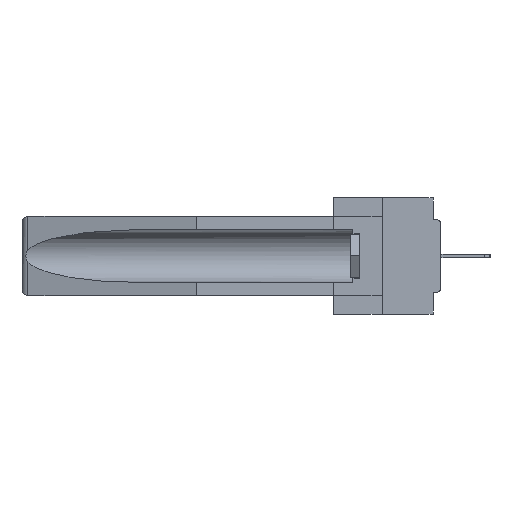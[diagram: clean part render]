
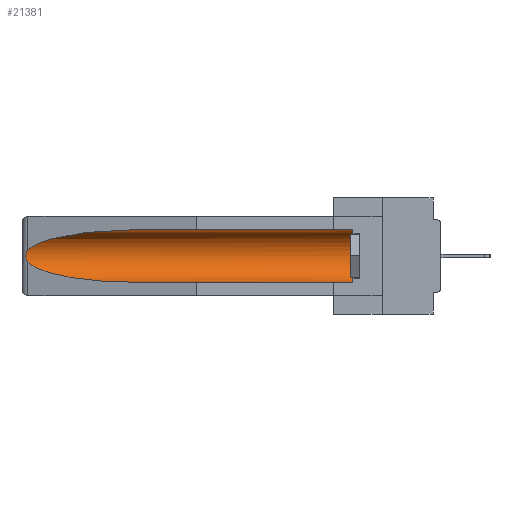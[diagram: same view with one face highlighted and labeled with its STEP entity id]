
A CAD part, left-side view. The second image highlights one B-rep face of the part: STEP entity #21381.
In plain terms, the highlighted cylindrical face has radius 2.857 mm (diameter 5.715 mm), a partial arc.
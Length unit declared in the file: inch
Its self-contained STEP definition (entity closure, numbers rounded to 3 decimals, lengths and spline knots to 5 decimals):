
#842 =( BOUNDED_CURVE ( )  B_SPLINE_CURVE ( 3, ( #7935, #8410, #2810, #5614 ),
 .UNSPECIFIED., .F., .F. ) 
 B_SPLINE_CURVE_WITH_KNOTS ( ( 4, 4 ),
 ( 0.1948, 1.5708 ),
 .UNSPECIFIED. ) 
 CURVE ( )  GEOMETRIC_REPRESENTATION_ITEM ( )  RATIONAL_B_SPLINE_CURVE ( ( 1., 0.848, 0.848, 1. ) ) 
 REPRESENTATION_ITEM ( '' )  );
#1557 = EDGE_CURVE ( 'NONE', #12987, #19888, #22805, .T. ) ;
#1878 = LINE ( 'NONE', #9308, #30999 ) ;
#2533 = CARTESIAN_POINT ( 'NONE',  ( 0.2675, 1.53308, -0.16763 ) ) ;
#2810 = CARTESIAN_POINT ( 'NONE',  ( 0.21114, 1.30732, -0.284 ) ) ;
#3015 = CARTESIAN_POINT ( 'NONE',  ( 0.26597, 1.5296, -0.19026 ) ) ;
#3927 = EDGE_LOOP ( 'NONE', ( #12949, #23673, #14191, #20234, #22389, #15519 ) ) ;
#4644 = EDGE_CURVE ( 'NONE', #16827, #7737, #842, .T. ) ;
#4791 = AXIS2_PLACEMENT_3D ( 'NONE', #25932, #20334, #13155 ) ;
#4849 = CARTESIAN_POINT ( 'NONE',  ( 0.26537, 1.52718, -0.19328 ) ) ;
#5614 = CARTESIAN_POINT ( 'NONE',  ( 0.155, 1.07973, -0.284 ) ) ;
#6526 =( BOUNDED_CURVE ( )  B_SPLINE_CURVE ( 3, ( #12414, #9428, #15060, #25206 ),
 .UNSPECIFIED., .F., .F. ) 
 B_SPLINE_CURVE_WITH_KNOTS ( ( 4, 4 ),
 ( 4.71239, 6.08839 ),
 .UNSPECIFIED. ) 
 CURVE ( )  GEOMETRIC_REPRESENTATION_ITEM ( )  RATIONAL_B_SPLINE_CURVE ( ( 1., 0.848, 0.848, 1. ) ) 
 REPRESENTATION_ITEM ( '' )  );
#7192 = DIRECTION ( 'NONE',  ( 0., 1., 0. ) ) ;
#7737 = VERTEX_POINT ( 'NONE', #19117 ) ;
#7935 = CARTESIAN_POINT ( 'NONE',  ( 0.26537, 1.52718, -0.19328 ) ) ;
#7988 = CARTESIAN_POINT ( 'NONE',  ( 0.2673, 1.53269, -0.17917 ) ) ;
#8410 = CARTESIAN_POINT ( 'NONE',  ( 0.25451, 1.48313, -0.24835 ) ) ;
#8423 = CARTESIAN_POINT ( 'NONE',  ( 0.155, -0.30754, -0.059 ) ) ;
#9062 = LINE ( 'NONE', #8423, #25898 ) ;
#9308 = CARTESIAN_POINT ( 'NONE',  ( 0.155, -0.30754, -0.284 ) ) ;
#9428 = CARTESIAN_POINT ( 'NONE',  ( 0.21114, 1.30732, -0.059 ) ) ;
#10642 = CARTESIAN_POINT ( 'NONE',  ( 0.26597, 1.52961, -0.15275 ) ) ;
#11055 = B_SPLINE_CURVE_WITH_KNOTS ( 'NONE', 3,
 ( #20769, #10642, #28203, #25419, #2533, #20602, #7988, #13277, #3015, #28362 ),
 .UNSPECIFIED., .F., .F.,
 ( 4, 2, 2, 2, 4 ),
 ( 0., 0.00029, 0.00058, 0.00087, 0.00117 ),
 .UNSPECIFIED. ) ;
#11084 = DIRECTION ( 'NONE',  ( 0., 1., 0. ) ) ;
#11542 = CARTESIAN_POINT ( 'NONE',  ( 0.26537, 1.52718, -0.14972 ) ) ;
#11875 = CARTESIAN_POINT ( 'NONE',  ( 0.155, 1.07973, -0.059 ) ) ;
#12414 = CARTESIAN_POINT ( 'NONE',  ( 0.155, 1.07973, -0.059 ) ) ;
#12949 = ORIENTED_EDGE ( 'NONE', *, *, #30258, .T. ) ;
#12987 = VERTEX_POINT ( 'NONE', #32319 ) ;
#13155 = DIRECTION ( 'NONE',  ( 0., 0., 1. ) ) ;
#13277 = CARTESIAN_POINT ( 'NONE',  ( 0.26655, 1.53094, -0.18657 ) ) ;
#14191 = ORIENTED_EDGE ( 'NONE', *, *, #4644, .T. ) ;
#14271 = DIRECTION ( 'NONE',  ( 0., 1., 0. ) ) ;
#14787 = CYLINDRICAL_SURFACE ( 'NONE', #23427, 0.1125 ) ;
#15060 = CARTESIAN_POINT ( 'NONE',  ( 0.25451, 1.48313, -0.09465 ) ) ;
#15519 = ORIENTED_EDGE ( 'NONE', *, *, #30442, .T. ) ;
#16827 = VERTEX_POINT ( 'NONE', #4849 ) ;
#19117 = CARTESIAN_POINT ( 'NONE',  ( 0.155, 1.07973, -0.284 ) ) ;
#19888 = VERTEX_POINT ( 'NONE', #31501 ) ;
#20234 = ORIENTED_EDGE ( 'NONE', *, *, #25627, .F. ) ;
#20334 = DIRECTION ( 'NONE',  ( 0., -1., 0. ) ) ;
#20602 = CARTESIAN_POINT ( 'NONE',  ( 0.2675, 1.53308, -0.17534 ) ) ;
#20769 = CARTESIAN_POINT ( 'NONE',  ( 0.26537, 1.52718, -0.14972 ) ) ;
#21381 = ADVANCED_FACE ( 'NONE', ( #22612 ), #14787, .F. ) ;
#21996 = VERTEX_POINT ( 'NONE', #11542 ) ;
#22389 = ORIENTED_EDGE ( 'NONE', *, *, #1557, .T. ) ;
#22612 = FACE_OUTER_BOUND ( 'NONE', #3927, .T. ) ;
#22805 = CIRCLE ( 'NONE', #4791, 0.1125 ) ;
#23427 = AXIS2_PLACEMENT_3D ( 'NONE', #32700, #7192, #24937 ) ;
#23673 = ORIENTED_EDGE ( 'NONE', *, *, #26920, .T. ) ;
#24937 = DIRECTION ( 'NONE',  ( 0., 0., 1. ) ) ;
#25206 = CARTESIAN_POINT ( 'NONE',  ( 0.26537, 1.52718, -0.14972 ) ) ;
#25419 = CARTESIAN_POINT ( 'NONE',  ( 0.2673, 1.5327, -0.16383 ) ) ;
#25627 = EDGE_CURVE ( 'NONE', #12987, #7737, #1878, .T. ) ;
#25898 = VECTOR ( 'NONE', #11084, 39.37008 ) ;
#25932 = CARTESIAN_POINT ( 'NONE',  ( 0.155, 0.126, -0.1715 ) ) ;
#26426 = VERTEX_POINT ( 'NONE', #11875 ) ;
#26920 = EDGE_CURVE ( 'NONE', #21996, #16827, #11055, .T. ) ;
#28203 = CARTESIAN_POINT ( 'NONE',  ( 0.26654, 1.53092, -0.15636 ) ) ;
#28362 = CARTESIAN_POINT ( 'NONE',  ( 0.26537, 1.52718, -0.19328 ) ) ;
#30258 = EDGE_CURVE ( 'NONE', #26426, #21996, #6526, .T. ) ;
#30442 = EDGE_CURVE ( 'NONE', #19888, #26426, #9062, .T. ) ;
#30999 = VECTOR ( 'NONE', #14271, 39.37008 ) ;
#31501 = CARTESIAN_POINT ( 'NONE',  ( 0.155, 0.126, -0.059 ) ) ;
#32319 = CARTESIAN_POINT ( 'NONE',  ( 0.155, 0.126, -0.284 ) ) ;
#32700 = CARTESIAN_POINT ( 'NONE',  ( 0.155, -0.30754, -0.1715 ) ) ;
